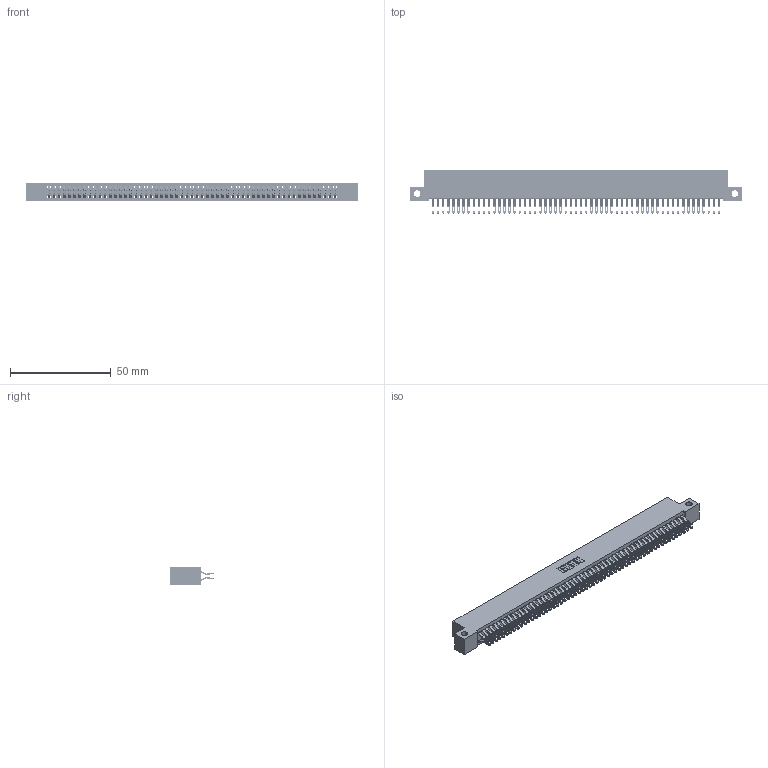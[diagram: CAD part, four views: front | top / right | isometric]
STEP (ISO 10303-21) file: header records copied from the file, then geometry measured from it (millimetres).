
FILE_DESCRIPTION (( 'STEP AP203' ), '1' );
FILE_NAME ('342-114-555-212.STEP', '2019-10-04T21:44:56', ( '' ), ( '' ), 'SwSTEP 2.0', 'SolidWorks 2016', '' );
FILE_SCHEMA (( 'CONFIG_CONTROL_DESIGN' ));
Length unit declared in the file: inch
Products named in the file (3): 342 Part_Side Mount; 345-292-001_555 Tail; 342-114-555-212
Assembly tree (115 placements, depth 2):
  342-114-555-212
    342 Part_Side Mount
    345-292-001_555 Tail  x114
Bounding box: 165.1 x 21.47 x 9.4 mm (x, y, z)
Volume: 15148.1 mm3; surface area: 25970.2 mm2
Topology: 115 solids, 115 shells, 6722 faces, 21161 edges, 14106 vertices
Faces by surface type: plane 3942, cylinder 2780
Entity records: 34927 total; most frequent: CARTESIAN_POINT 5804, ORIENTED_EDGE 5710, DIRECTION 4903, EDGE_CURVE 2855, LINE 2707, VECTOR 2707, VERTEX_POINT 1902, AXIS2_PLACEMENT_3D 1098
